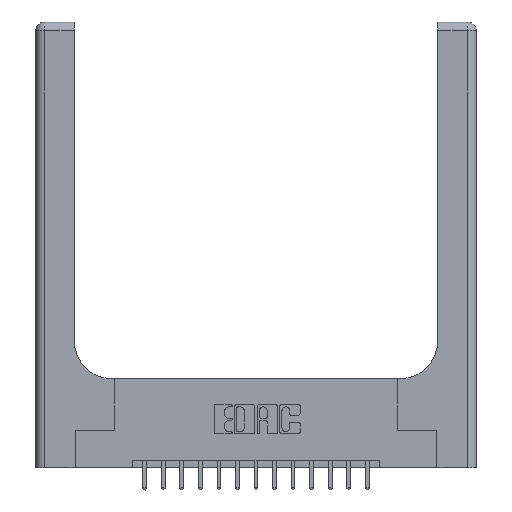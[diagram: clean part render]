
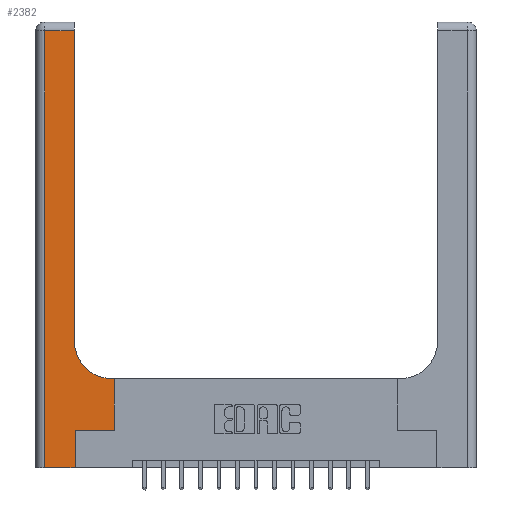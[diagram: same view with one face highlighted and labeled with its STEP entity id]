
A CAD part, top view. The second image highlights one B-rep face of the part: STEP entity #2382.
In plain terms, the highlighted planar face has unit normal (0, 0, 1).
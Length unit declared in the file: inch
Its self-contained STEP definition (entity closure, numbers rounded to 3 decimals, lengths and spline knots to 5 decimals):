
#14 = VERTEX_POINT ( 'NONE', #16779 ) ;
#237 = CIRCLE ( 'NONE', #8325, 0.25 ) ;
#238 = DIRECTION ( 'NONE',  ( -1., 0., 0. ) ) ;
#260 = VECTOR ( 'NONE', #2571, 39.37008 ) ;
#567 = VECTOR ( 'NONE', #14324, 39.37008 ) ;
#634 = EDGE_CURVE ( 'NONE', #13374, #12021, #12208, .T. ) ;
#740 = ORIENTED_EDGE ( 'NONE', *, *, #14607, .T. ) ;
#964 = VECTOR ( 'NONE', #9341, 39.37008 ) ;
#1064 = CARTESIAN_POINT ( 'NONE',  ( 0.265, 0., 0.37 ) ) ;
#1222 = EDGE_CURVE ( 'NONE', #13966, #14, #237, .T. ) ;
#1746 = DIRECTION ( 'NONE',  ( -1., 0., 0. ) ) ;
#1922 = LINE ( 'NONE', #6616, #10654 ) ;
#1976 = LINE ( 'NONE', #10750, #11107 ) ;
#2382 = ADVANCED_FACE ( 'NONE', ( #7386 ), #9800, .F. ) ;
#2571 = DIRECTION ( 'NONE',  ( 0., 1., 0. ) ) ;
#2606 = VERTEX_POINT ( 'NONE', #13137 ) ;
#2670 = LINE ( 'NONE', #7173, #16678 ) ;
#2700 = LINE ( 'NONE', #5115, #9684 ) ;
#2702 = ORIENTED_EDGE ( 'NONE', *, *, #3851, .T. ) ;
#3305 = CARTESIAN_POINT ( 'NONE',  ( 0.51, 0.85, 0.37 ) ) ;
#3479 = VERTEX_POINT ( 'NONE', #1064 ) ;
#3529 = DIRECTION ( 'NONE',  ( 0., -1., 0. ) ) ;
#3561 = CARTESIAN_POINT ( 'NONE',  ( 0.26, 2.94, 0.37 ) ) ;
#3585 = ORIENTED_EDGE ( 'NONE', *, *, #634, .T. ) ;
#3851 = EDGE_CURVE ( 'NONE', #16061, #12867, #2670, .T. ) ;
#4340 = ORIENTED_EDGE ( 'NONE', *, *, #8486, .T. ) ;
#4506 = DIRECTION ( 'NONE',  ( 1., 0., 0. ) ) ;
#4682 = EDGE_CURVE ( 'NONE', #14, #16061, #1976, .T. ) ;
#5115 = CARTESIAN_POINT ( 'NONE',  ( 0.265, 0., 0.37 ) ) ;
#5318 = DIRECTION ( 'NONE',  ( 0., 1., 0. ) ) ;
#6368 = ORIENTED_EDGE ( 'NONE', *, *, #4682, .T. ) ;
#6465 = VECTOR ( 'NONE', #3529, 39.37008 ) ;
#6616 = CARTESIAN_POINT ( 'NONE',  ( 0., 0., 0.37 ) ) ;
#7073 = DIRECTION ( 'NONE',  ( 0., 0., -1. ) ) ;
#7173 = CARTESIAN_POINT ( 'NONE',  ( 0., 2.94, 0.37 ) ) ;
#7386 = FACE_OUTER_BOUND ( 'NONE', #10223, .T. ) ;
#7738 = ORIENTED_EDGE ( 'NONE', *, *, #11765, .T. ) ;
#7813 = CARTESIAN_POINT ( 'NONE',  ( 0.265, 0.25, 0.37 ) ) ;
#8325 = AXIS2_PLACEMENT_3D ( 'NONE', #3305, #12807, #4506 ) ;
#8386 = ORIENTED_EDGE ( 'NONE', *, *, #9002, .T. ) ;
#8486 = EDGE_CURVE ( 'NONE', #12021, #13966, #10581, .T. ) ;
#8768 = EDGE_CURVE ( 'NONE', #12867, #2606, #12890, .T. ) ;
#9002 = EDGE_CURVE ( 'NONE', #3479, #13713, #2700, .T. ) ;
#9341 = DIRECTION ( 'NONE',  ( 1., 0., 0. ) ) ;
#9684 = VECTOR ( 'NONE', #13228, 39.37008 ) ;
#9800 = PLANE ( 'NONE',  #16178 ) ;
#10080 = ORIENTED_EDGE ( 'NONE', *, *, #8768, .T. ) ;
#10119 = CARTESIAN_POINT ( 'NONE',  ( 0.06, 2.94, 0.37 ) ) ;
#10223 = EDGE_LOOP ( 'NONE', ( #6368, #2702, #10080, #740, #8386, #7738, #3585, #4340, #11017 ) ) ;
#10230 = CARTESIAN_POINT ( 'NONE',  ( 0.26, 0.6, 0.37 ) ) ;
#10581 = LINE ( 'NONE', #10230, #567 ) ;
#10654 = VECTOR ( 'NONE', #14709, 39.37008 ) ;
#10750 = CARTESIAN_POINT ( 'NONE',  ( 0.26, 3., 0.37 ) ) ;
#10757 = CARTESIAN_POINT ( 'NONE',  ( 0.528, 0.25, 0.37 ) ) ;
#11017 = ORIENTED_EDGE ( 'NONE', *, *, #1222, .T. ) ;
#11107 = VECTOR ( 'NONE', #5318, 39.37008 ) ;
#11288 = CARTESIAN_POINT ( 'NONE',  ( 0.528, 0.6, 0.37 ) ) ;
#11765 = EDGE_CURVE ( 'NONE', #13713, #13374, #16916, .T. ) ;
#12021 = VERTEX_POINT ( 'NONE', #11288 ) ;
#12208 = LINE ( 'NONE', #17407, #260 ) ;
#12807 = DIRECTION ( 'NONE',  ( 0., 0., -1. ) ) ;
#12867 = VERTEX_POINT ( 'NONE', #10119 ) ;
#12890 = LINE ( 'NONE', #17080, #6465 ) ;
#13137 = CARTESIAN_POINT ( 'NONE',  ( 0.06, 0., 0.37 ) ) ;
#13228 = DIRECTION ( 'NONE',  ( 0., 1., 0. ) ) ;
#13374 = VERTEX_POINT ( 'NONE', #10757 ) ;
#13592 = CARTESIAN_POINT ( 'NONE',  ( 0.51, 0.6, 0.37 ) ) ;
#13713 = VERTEX_POINT ( 'NONE', #14318 ) ;
#13966 = VERTEX_POINT ( 'NONE', #13592 ) ;
#14318 = CARTESIAN_POINT ( 'NONE',  ( 0.265, 0.25, 0.37 ) ) ;
#14324 = DIRECTION ( 'NONE',  ( -1., 0., 0. ) ) ;
#14607 = EDGE_CURVE ( 'NONE', #2606, #3479, #1922, .T. ) ;
#14709 = DIRECTION ( 'NONE',  ( 1., 0., 0. ) ) ;
#15237 = CARTESIAN_POINT ( 'NONE',  ( 0., 3., 0.37 ) ) ;
#16061 = VERTEX_POINT ( 'NONE', #3561 ) ;
#16178 = AXIS2_PLACEMENT_3D ( 'NONE', #15237, #7073, #238 ) ;
#16678 = VECTOR ( 'NONE', #1746, 39.37008 ) ;
#16779 = CARTESIAN_POINT ( 'NONE',  ( 0.26, 0.85, 0.37 ) ) ;
#16916 = LINE ( 'NONE', #7813, #964 ) ;
#17080 = CARTESIAN_POINT ( 'NONE',  ( 0.06, 3., 0.37 ) ) ;
#17407 = CARTESIAN_POINT ( 'NONE',  ( 0.528, 0.25, 0.37 ) ) ;
